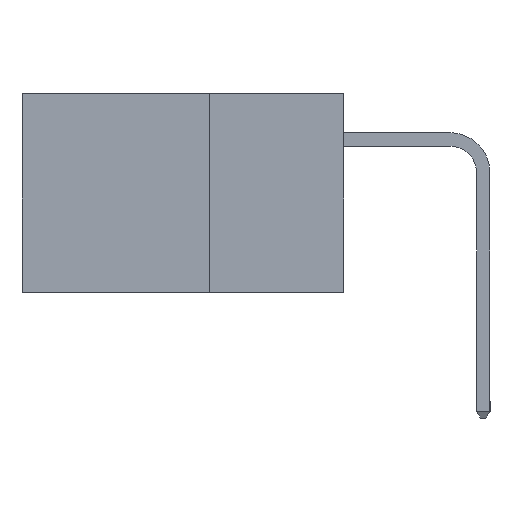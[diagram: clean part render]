
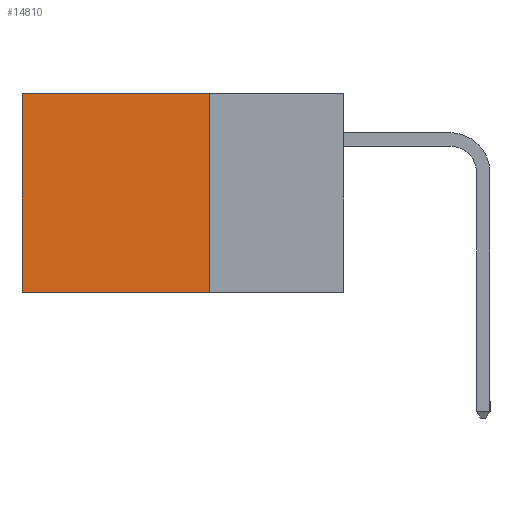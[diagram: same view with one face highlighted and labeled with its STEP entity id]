
A CAD part, left-side view. The second image highlights one B-rep face of the part: STEP entity #14810.
In plain terms, the highlighted planar face has unit normal (-1, 0, 0).
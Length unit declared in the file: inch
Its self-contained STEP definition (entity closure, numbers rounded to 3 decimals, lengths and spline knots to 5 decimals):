
#311 = LINE ( 'NONE', #3388, #13759 ) ;
#728 = DIRECTION ( 'NONE',  ( 0., 0., -1. ) ) ;
#1236 = VECTOR ( 'NONE', #15557, 39.37008 ) ;
#2460 = EDGE_CURVE ( 'NONE', #13602, #10160, #10466, .T. ) ;
#2530 = DIRECTION ( 'NONE',  ( 0., 0., -1. ) ) ;
#2677 = CARTESIAN_POINT ( 'NONE',  ( 0.2615, 0.6, -0.37 ) ) ;
#2685 = CARTESIAN_POINT ( 'NONE',  ( 0.2615, 0.25, -0.37 ) ) ;
#3198 = EDGE_CURVE ( 'NONE', #6633, #12368, #9865, .T. ) ;
#3388 = CARTESIAN_POINT ( 'NONE',  ( 0.2615, 0.25, -0.37 ) ) ;
#3695 = CARTESIAN_POINT ( 'NONE',  ( 0.2615, 0.25, -0.37 ) ) ;
#3787 = EDGE_CURVE ( 'NONE', #6633, #13602, #8238, .T. ) ;
#3833 = EDGE_CURVE ( 'NONE', #12368, #10160, #311, .T. ) ;
#3969 = ORIENTED_EDGE ( 'NONE', *, *, #2460, .T. ) ;
#4085 = DIRECTION ( 'NONE',  ( 0., 0., -1. ) ) ;
#4535 = CARTESIAN_POINT ( 'NONE',  ( 0.2615, 0.25, 0. ) ) ;
#6098 = CARTESIAN_POINT ( 'NONE',  ( 0.2615, 0.6, -0.37 ) ) ;
#6331 = AXIS2_PLACEMENT_3D ( 'NONE', #2685, #11653, #4085 ) ;
#6633 = VERTEX_POINT ( 'NONE', #4535 ) ;
#6884 = ORIENTED_EDGE ( 'NONE', *, *, #3198, .F. ) ;
#7125 = VECTOR ( 'NONE', #2530, 39.37008 ) ;
#8238 = LINE ( 'NONE', #8262, #1236 ) ;
#8262 = CARTESIAN_POINT ( 'NONE',  ( 0.2615, 0.25, 0. ) ) ;
#9865 = LINE ( 'NONE', #3695, #15997 ) ;
#10160 = VERTEX_POINT ( 'NONE', #6098 ) ;
#10387 = PLANE ( 'NONE',  #6331 ) ;
#10466 = LINE ( 'NONE', #2677, #7125 ) ;
#10505 = FACE_OUTER_BOUND ( 'NONE', #13971, .T. ) ;
#11653 = DIRECTION ( 'NONE',  ( 1., 0., 0. ) ) ;
#12368 = VERTEX_POINT ( 'NONE', #13918 ) ;
#13280 = ORIENTED_EDGE ( 'NONE', *, *, #3787, .T. ) ;
#13602 = VERTEX_POINT ( 'NONE', #16352 ) ;
#13759 = VECTOR ( 'NONE', #14266, 39.37008 ) ;
#13918 = CARTESIAN_POINT ( 'NONE',  ( 0.2615, 0.25, -0.37 ) ) ;
#13971 = EDGE_LOOP ( 'NONE', ( #3969, #15425, #6884, #13280 ) ) ;
#14266 = DIRECTION ( 'NONE',  ( 0., 1., 0. ) ) ;
#14810 = ADVANCED_FACE ( 'NONE', ( #10505 ), #10387, .F. ) ;
#15425 = ORIENTED_EDGE ( 'NONE', *, *, #3833, .F. ) ;
#15557 = DIRECTION ( 'NONE',  ( 0., 1., 0. ) ) ;
#15997 = VECTOR ( 'NONE', #728, 39.37008 ) ;
#16352 = CARTESIAN_POINT ( 'NONE',  ( 0.2615, 0.6, 0. ) ) ;
